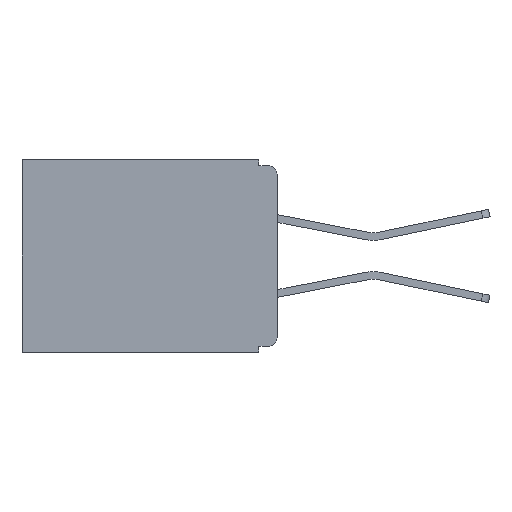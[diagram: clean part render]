
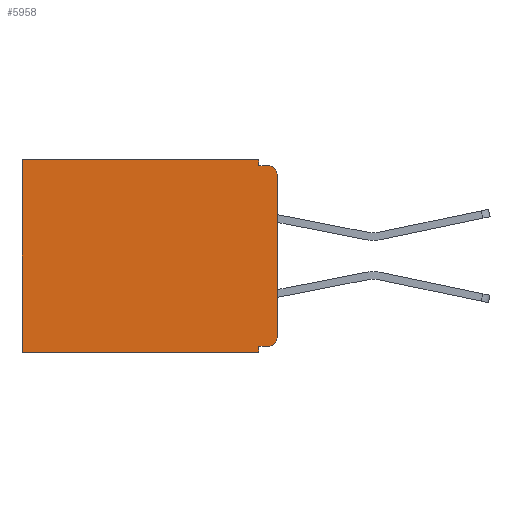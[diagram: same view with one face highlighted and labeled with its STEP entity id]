
A CAD part, left-side view. The second image highlights one B-rep face of the part: STEP entity #5958.
In plain terms, the highlighted planar face has unit normal (-1, 0, 0).
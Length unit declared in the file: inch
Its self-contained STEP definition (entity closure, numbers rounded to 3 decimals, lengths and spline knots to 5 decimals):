
#23 = EDGE_CURVE ( 'NONE', #12133, #21616, #15791, .T. ) ;
#81 = CARTESIAN_POINT ( 'NONE',  ( 0.3, 0.437, 0. ) ) ;
#574 = CARTESIAN_POINT ( 'NONE',  ( 0.3, 0.015, -0.01 ) ) ;
#1296 = CARTESIAN_POINT ( 'NONE',  ( 0.3, 0.015, -0.025 ) ) ;
#1573 = CARTESIAN_POINT ( 'NONE',  ( 0.3, 0.437, -0.33 ) ) ;
#2071 = DIRECTION ( 'NONE',  ( 0., -1., 0. ) ) ;
#2233 = ORIENTED_EDGE ( 'NONE', *, *, #23, .T. ) ;
#2469 = CARTESIAN_POINT ( 'NONE',  ( 0.3, 0.015, -0.305 ) ) ;
#2551 = ORIENTED_EDGE ( 'NONE', *, *, #17377, .T. ) ;
#2637 = DIRECTION ( 'NONE',  ( 0., 0., -1. ) ) ;
#2905 = VERTEX_POINT ( 'NONE', #15451 ) ;
#3011 = EDGE_CURVE ( 'NONE', #18667, #14614, #7848, .T. ) ;
#3071 = CARTESIAN_POINT ( 'NONE',  ( 0.3, 0., -0.32 ) ) ;
#3891 = DIRECTION ( 'NONE',  ( 1., 0., 0. ) ) ;
#4217 = AXIS2_PLACEMENT_3D ( 'NONE', #23912, #3891, #2637 ) ;
#4701 = ORIENTED_EDGE ( 'NONE', *, *, #24101, .F. ) ;
#5694 = VECTOR ( 'NONE', #19618, 39.37008 ) ;
#5958 = ADVANCED_FACE ( 'NONE', ( #19069 ), #16063, .F. ) ;
#6215 = VECTOR ( 'NONE', #2071, 39.37008 ) ;
#6611 = LINE ( 'NONE', #23224, #22518 ) ;
#7193 = DIRECTION ( 'NONE',  ( 0., 0., -1. ) ) ;
#7348 = EDGE_CURVE ( 'NONE', #12133, #18333, #18340, .T. ) ;
#7546 = DIRECTION ( 'NONE',  ( -1., 0., 0. ) ) ;
#7848 = CIRCLE ( 'NONE', #22516, 0.015 ) ;
#7868 = LINE ( 'NONE', #13217, #18297 ) ;
#8211 = ORIENTED_EDGE ( 'NONE', *, *, #14521, .F. ) ;
#8292 = CARTESIAN_POINT ( 'NONE',  ( 0.3, 0.031, -0.33 ) ) ;
#8738 = AXIS2_PLACEMENT_3D ( 'NONE', #2469, #7546, #7193 ) ;
#8777 = DIRECTION ( 'NONE',  ( 0., 0., -1. ) ) ;
#9022 = DIRECTION ( 'NONE',  ( 0., 0., -1. ) ) ;
#9031 = LINE ( 'NONE', #16082, #20116 ) ;
#9525 = ORIENTED_EDGE ( 'NONE', *, *, #14774, .T. ) ;
#10871 = VERTEX_POINT ( 'NONE', #15950 ) ;
#11097 = VERTEX_POINT ( 'NONE', #20733 ) ;
#11265 = LINE ( 'NONE', #13378, #5694 ) ;
#11336 = ORIENTED_EDGE ( 'NONE', *, *, #15920, .F. ) ;
#11746 = VECTOR ( 'NONE', #12198, 39.37008 ) ;
#12006 = VECTOR ( 'NONE', #9022, 39.37008 ) ;
#12133 = VERTEX_POINT ( 'NONE', #26231 ) ;
#12198 = DIRECTION ( 'NONE',  ( 0., 0., -1. ) ) ;
#12404 = LINE ( 'NONE', #1573, #11746 ) ;
#13217 = CARTESIAN_POINT ( 'NONE',  ( 0.3, 0.031, -0.33 ) ) ;
#13378 = CARTESIAN_POINT ( 'NONE',  ( 0.3, 0., -0.33 ) ) ;
#13828 = CARTESIAN_POINT ( 'NONE',  ( 0.3, 0., -0.305 ) ) ;
#14180 = ORIENTED_EDGE ( 'NONE', *, *, #7348, .F. ) ;
#14365 = EDGE_CURVE ( 'NONE', #10871, #14614, #17323, .T. ) ;
#14521 = EDGE_CURVE ( 'NONE', #18333, #14835, #7868, .T. ) ;
#14614 = VERTEX_POINT ( 'NONE', #574 ) ;
#14774 = EDGE_CURVE ( 'NONE', #19218, #11097, #12404, .T. ) ;
#14835 = VERTEX_POINT ( 'NONE', #8292 ) ;
#15171 = ORIENTED_EDGE ( 'NONE', *, *, #14365, .F. ) ;
#15221 = CARTESIAN_POINT ( 'NONE',  ( 0.3, 0.031, 0. ) ) ;
#15297 = DIRECTION ( 'NONE',  ( 0., 0., -1. ) ) ;
#15451 = CARTESIAN_POINT ( 'NONE',  ( 0.3, 0.031, 0. ) ) ;
#15791 = CIRCLE ( 'NONE', #8738, 0.015 ) ;
#15920 = EDGE_CURVE ( 'NONE', #2905, #10871, #17573, .T. ) ;
#15950 = CARTESIAN_POINT ( 'NONE',  ( 0.3, 0.031, -0.01 ) ) ;
#16018 = ORIENTED_EDGE ( 'NONE', *, *, #3011, .T. ) ;
#16063 = PLANE ( 'NONE',  #4217 ) ;
#16082 = CARTESIAN_POINT ( 'NONE',  ( 0.3, 0., 0. ) ) ;
#16703 = DIRECTION ( 'NONE',  ( -1., 0., 0. ) ) ;
#16866 = CARTESIAN_POINT ( 'NONE',  ( 0.3, 0., -0.01 ) ) ;
#17323 = LINE ( 'NONE', #16866, #6215 ) ;
#17377 = EDGE_CURVE ( 'NONE', #2905, #19218, #9031, .T. ) ;
#17573 = LINE ( 'NONE', #15221, #12006 ) ;
#18179 = DIRECTION ( 'NONE',  ( 0., 1., 0. ) ) ;
#18245 = ORIENTED_EDGE ( 'NONE', *, *, #19923, .F. ) ;
#18297 = VECTOR ( 'NONE', #15297, 39.37008 ) ;
#18333 = VERTEX_POINT ( 'NONE', #22077 ) ;
#18340 = LINE ( 'NONE', #3071, #23704 ) ;
#18667 = VERTEX_POINT ( 'NONE', #25440 ) ;
#19069 = FACE_OUTER_BOUND ( 'NONE', #20412, .T. ) ;
#19218 = VERTEX_POINT ( 'NONE', #81 ) ;
#19618 = DIRECTION ( 'NONE',  ( 0., 1., 0. ) ) ;
#19891 = DIRECTION ( 'NONE',  ( 0., 1., 0. ) ) ;
#19923 = EDGE_CURVE ( 'NONE', #18667, #21616, #6611, .T. ) ;
#20116 = VECTOR ( 'NONE', #18179, 39.37008 ) ;
#20412 = EDGE_LOOP ( 'NONE', ( #18245, #16018, #15171, #11336, #2551, #9525, #4701, #8211, #14180, #2233 ) ) ;
#20733 = CARTESIAN_POINT ( 'NONE',  ( 0.3, 0.437, -0.33 ) ) ;
#21616 = VERTEX_POINT ( 'NONE', #13828 ) ;
#21623 = DIRECTION ( 'NONE',  ( 0., 0., -1. ) ) ;
#22077 = CARTESIAN_POINT ( 'NONE',  ( 0.3, 0.031, -0.32 ) ) ;
#22516 = AXIS2_PLACEMENT_3D ( 'NONE', #1296, #16703, #21623 ) ;
#22518 = VECTOR ( 'NONE', #8777, 39.37008 ) ;
#23224 = CARTESIAN_POINT ( 'NONE',  ( 0.3, 0., -0.33 ) ) ;
#23704 = VECTOR ( 'NONE', #19891, 39.37008 ) ;
#23912 = CARTESIAN_POINT ( 'NONE',  ( 0.3, 0., -0.33 ) ) ;
#24101 = EDGE_CURVE ( 'NONE', #14835, #11097, #11265, .T. ) ;
#25440 = CARTESIAN_POINT ( 'NONE',  ( 0.3, 0., -0.025 ) ) ;
#26231 = CARTESIAN_POINT ( 'NONE',  ( 0.3, 0.015, -0.32 ) ) ;
